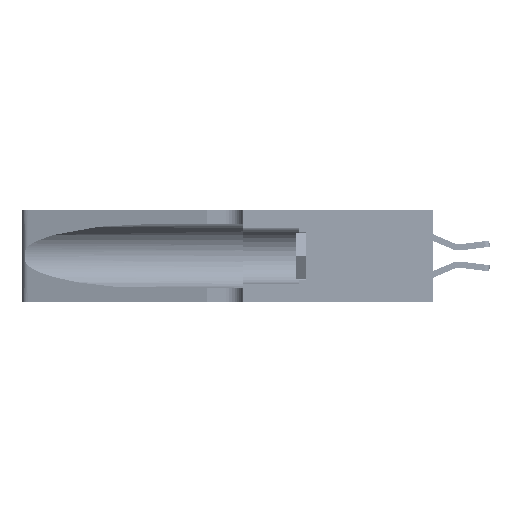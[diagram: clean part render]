
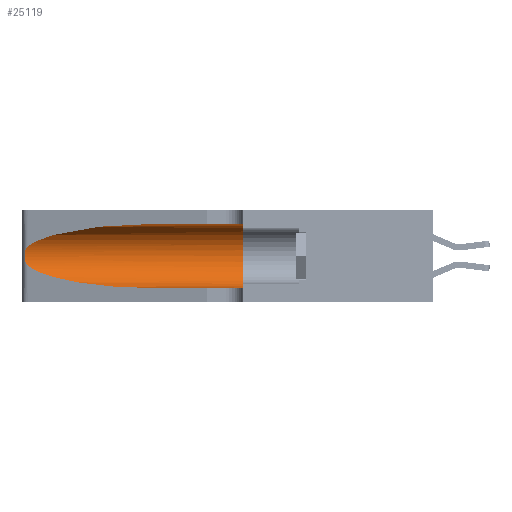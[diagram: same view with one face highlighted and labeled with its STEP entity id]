
A CAD part, left-side view. The second image highlights one B-rep face of the part: STEP entity #25119.
In plain terms, the highlighted cylindrical face has radius 3.308 mm (diameter 6.617 mm), a partial arc.
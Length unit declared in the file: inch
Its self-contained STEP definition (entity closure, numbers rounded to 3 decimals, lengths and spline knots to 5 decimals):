
#1172 = CARTESIAN_POINT ( 'NONE',  ( 0.2373, 1.15595, 0.28018 ) ) ;
#1663 = CARTESIAN_POINT ( 'NONE',  ( 0.1305, 0.35, 0.05475 ) ) ;
#1770 = VERTEX_POINT ( 'NONE', #25931 ) ;
#1993 = CARTESIAN_POINT ( 'NONE',  ( 0.25787, 1.23484, 0.2124 ) ) ;
#2520 = ORIENTED_EDGE ( 'NONE', *, *, #29621, .T. ) ;
#2550 = VERTEX_POINT ( 'NONE', #25192 ) ;
#2698 = DIRECTION ( 'NONE',  ( 0., -1., 0. ) ) ;
#4576 = CARTESIAN_POINT ( 'NONE',  ( 0.1305, 1.61858, 0.31525 ) ) ;
#5155 = CARTESIAN_POINT ( 'NONE',  ( 0.1305, 0.72297, 0.31525 ) ) ;
#5168 = EDGE_CURVE ( 'NONE', #7400, #1770, #35991, .T. ) ;
#5247 = LINE ( 'NONE', #11600, #31109 ) ;
#5632 = LINE ( 'NONE', #4576, #22804 ) ;
#6938 = CARTESIAN_POINT ( 'NONE',  ( 0.2373, 1.15595, 0.08982 ) ) ;
#6996 = EDGE_CURVE ( 'NONE', #2550, #20404, #35836, .T. ) ;
#7400 = VERTEX_POINT ( 'NONE', #24371 ) ;
#7641 = VERTEX_POINT ( 'NONE', #10542 ) ;
#9325 = CARTESIAN_POINT ( 'NONE',  ( 0.1305, 0.35, 0.185 ) ) ;
#9401 = EDGE_CURVE ( 'NONE', #34212, #7641, #26388, .T. ) ;
#10459 = CARTESIAN_POINT ( 'NONE',  ( 0.18966, 0.96281, 0.31525 ) ) ;
#10542 = CARTESIAN_POINT ( 'NONE',  ( 0.25487, 1.22718, 0.22369 ) ) ;
#10716 = DIRECTION ( 'NONE',  ( 0., 0., -1. ) ) ;
#10906 = EDGE_CURVE ( 'NONE', #7641, #7400, #13312, .T. ) ;
#11186 = ORIENTED_EDGE ( 'NONE', *, *, #5168, .T. ) ;
#11302 = CARTESIAN_POINT ( 'NONE',  ( 0.25555, 1.22994, 0.2215 ) ) ;
#11321 = DIRECTION ( 'NONE',  ( 0., 1., 0. ) ) ;
#11571 = CARTESIAN_POINT ( 'NONE',  ( 0.26075, 1.23896, 0.178 ) ) ;
#11600 = CARTESIAN_POINT ( 'NONE',  ( 0.1305, 1.61858, 0.05475 ) ) ;
#12345 = DIRECTION ( 'NONE',  ( 0., 0., 1. ) ) ;
#12917 = CYLINDRICAL_SURFACE ( 'NONE', #32964, 0.13025 ) ;
#13312 = B_SPLINE_CURVE_WITH_KNOTS ( 'NONE', 3,
 ( #37601, #11302, #31971, #1993, #16897, #26330, #21427, #11571, #38119, #26455, #18208, #36289, #36670, #36427 ),
 .UNSPECIFIED., .F., .F.,
 ( 4, 2, 2, 2, 2, 2, 4 ),
 ( 0., 0.00027, 0.00053, 0.00107, 0.0016, 0.00187, 0.00214 ),
 .UNSPECIFIED. ) ;
#13571 = EDGE_CURVE ( 'NONE', #34212, #2550, #5632, .T. ) ;
#15774 = CARTESIAN_POINT ( 'NONE',  ( 0.1305, 0.72297, 0.05475 ) ) ;
#16897 = CARTESIAN_POINT ( 'NONE',  ( 0.25854, 1.2359, 0.20912 ) ) ;
#17625 = ORIENTED_EDGE ( 'NONE', *, *, #6996, .F. ) ;
#17825 = ORIENTED_EDGE ( 'NONE', *, *, #10906, .T. ) ;
#18208 = CARTESIAN_POINT ( 'NONE',  ( 0.25789, 1.23486, 0.15765 ) ) ;
#18532 = CARTESIAN_POINT ( 'NONE',  ( 0.25487, 1.22718, 0.14631 ) ) ;
#19603 = DIRECTION ( 'NONE',  ( 0., -1., 0. ) ) ;
#20286 = EDGE_LOOP ( 'NONE', ( #22238, #17825, #11186, #2520, #17625, #30046 ) ) ;
#20404 = VERTEX_POINT ( 'NONE', #1663 ) ;
#21427 = CARTESIAN_POINT ( 'NONE',  ( 0.26075, 1.23896, 0.19203 ) ) ;
#22238 = ORIENTED_EDGE ( 'NONE', *, *, #9401, .T. ) ;
#22296 = CARTESIAN_POINT ( 'NONE',  ( 0.1305, 0.72297, 0.31525 ) ) ;
#22804 = VECTOR ( 'NONE', #28107, 39.37008 ) ;
#22919 = CARTESIAN_POINT ( 'NONE',  ( 0.25487, 1.22718, 0.22369 ) ) ;
#23587 = FACE_OUTER_BOUND ( 'NONE', #20286, .T. ) ;
#24371 = CARTESIAN_POINT ( 'NONE',  ( 0.25487, 1.22718, 0.14631 ) ) ;
#25119 = ADVANCED_FACE ( 'NONE', ( #23587 ), #12917, .F. ) ;
#25192 = CARTESIAN_POINT ( 'NONE',  ( 0.1305, 0.35, 0.31525 ) ) ;
#25931 = CARTESIAN_POINT ( 'NONE',  ( 0.1305, 0.72297, 0.05475 ) ) ;
#26207 = AXIS2_PLACEMENT_3D ( 'NONE', #9325, #11321, #12345 ) ;
#26330 = CARTESIAN_POINT ( 'NONE',  ( 0.26018, 1.23835, 0.19895 ) ) ;
#26388 =( BOUNDED_CURVE ( )  B_SPLINE_CURVE ( 3, ( #22296, #10459, #1172, #22919 ),
 .UNSPECIFIED., .F., .T. ) 
 B_SPLINE_CURVE_WITH_KNOTS ( ( 4, 4 ),
 ( 1.5708, 2.84003 ),
 .UNSPECIFIED. ) 
 CURVE ( )  GEOMETRIC_REPRESENTATION_ITEM ( )  RATIONAL_B_SPLINE_CURVE ( ( 1., 0.87, 0.87, 1. ) ) 
 REPRESENTATION_ITEM ( '' )  );
#26455 = CARTESIAN_POINT ( 'NONE',  ( 0.25856, 1.23593, 0.16098 ) ) ;
#28107 = DIRECTION ( 'NONE',  ( 0., -1., 0. ) ) ;
#29621 = EDGE_CURVE ( 'NONE', #1770, #20404, #5247, .T. ) ;
#30046 = ORIENTED_EDGE ( 'NONE', *, *, #13571, .F. ) ;
#31109 = VECTOR ( 'NONE', #2698, 39.37008 ) ;
#31971 = CARTESIAN_POINT ( 'NONE',  ( 0.25639, 1.23184, 0.21858 ) ) ;
#32964 = AXIS2_PLACEMENT_3D ( 'NONE', #37159, #19603, #10716 ) ;
#33427 = CARTESIAN_POINT ( 'NONE',  ( 0.18966, 0.96281, 0.05475 ) ) ;
#34212 = VERTEX_POINT ( 'NONE', #5155 ) ;
#35836 = CIRCLE ( 'NONE', #26207, 0.13025 ) ;
#35991 =( BOUNDED_CURVE ( )  B_SPLINE_CURVE ( 3, ( #18532, #6938, #33427, #15774 ),
 .UNSPECIFIED., .F., .T. ) 
 B_SPLINE_CURVE_WITH_KNOTS ( ( 4, 4 ),
 ( 3.44316, 4.71239 ),
 .UNSPECIFIED. ) 
 CURVE ( )  GEOMETRIC_REPRESENTATION_ITEM ( )  RATIONAL_B_SPLINE_CURVE ( ( 1., 0.87, 0.87, 1. ) ) 
 REPRESENTATION_ITEM ( '' )  );
#36289 = CARTESIAN_POINT ( 'NONE',  ( 0.25639, 1.23186, 0.15144 ) ) ;
#36427 = CARTESIAN_POINT ( 'NONE',  ( 0.25487, 1.22718, 0.14631 ) ) ;
#36670 = CARTESIAN_POINT ( 'NONE',  ( 0.25555, 1.22993, 0.14849 ) ) ;
#37159 = CARTESIAN_POINT ( 'NONE',  ( 0.1305, 1.61858, 0.185 ) ) ;
#37601 = CARTESIAN_POINT ( 'NONE',  ( 0.25487, 1.22718, 0.22369 ) ) ;
#38119 = CARTESIAN_POINT ( 'NONE',  ( 0.26017, 1.23833, 0.17102 ) ) ;
